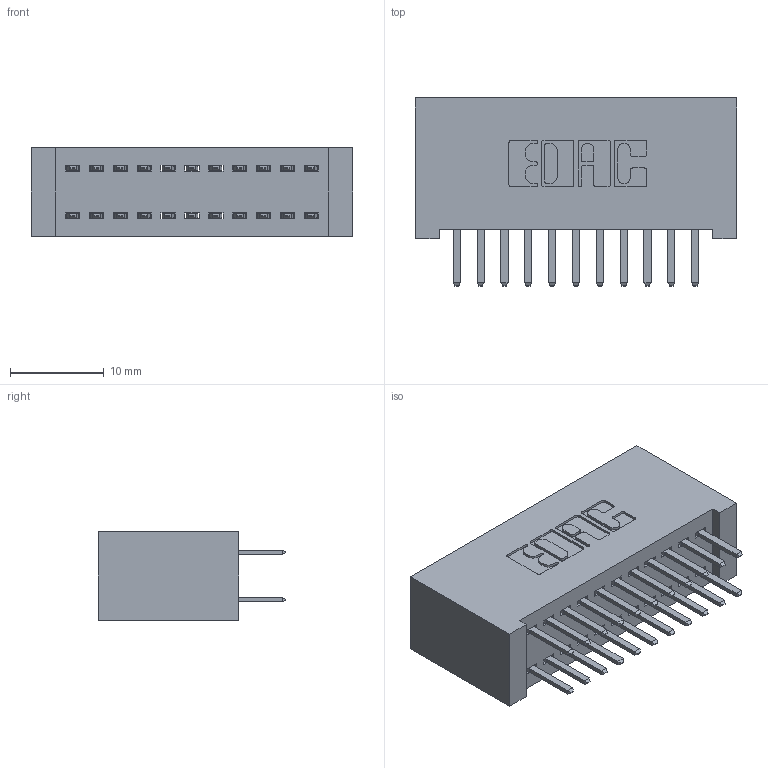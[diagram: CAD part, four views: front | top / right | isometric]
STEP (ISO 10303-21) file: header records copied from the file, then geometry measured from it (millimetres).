
FILE_DESCRIPTION (( 'STEP AP203' ), '1' );
FILE_NAME ('392-022-520-201.STEP', '2018-08-15T12:27:02', ( '' ), ( '' ), 'SwSTEP 2.0', 'SolidWorks 2016', '' );
FILE_SCHEMA (( 'CONFIG_CONTROL_DESIGN' ));
Length unit declared in the file: inch
Products named in the file (3): 342 Part_Lugless; 345-292-001_345-293-120; 392-022-520-201
Assembly tree (23 placements, depth 2):
  392-022-520-201
    342 Part_Lugless
    345-292-001_345-293-120  x22
Bounding box: 34.19 x 20.02 x 9.4 mm (x, y, z)
Volume: 3354.9 mm3; surface area: 5120.5 mm2
Topology: 23 solids, 23 shells, 1334 faces, 3861 edges, 2514 vertices
Faces by surface type: plane 898, cylinder 436
Entity records: 10791 total; most frequent: CARTESIAN_POINT 1834, ORIENTED_EDGE 1758, DIRECTION 1603, EDGE_CURVE 879, LINE 755, VECTOR 755, VERTEX_POINT 582, AXIS2_PLACEMENT_3D 424
